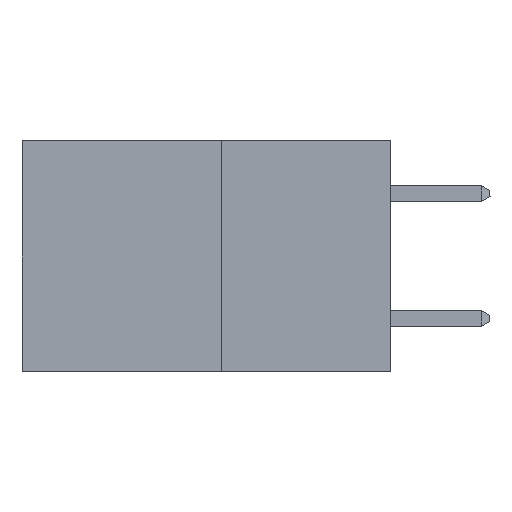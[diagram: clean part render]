
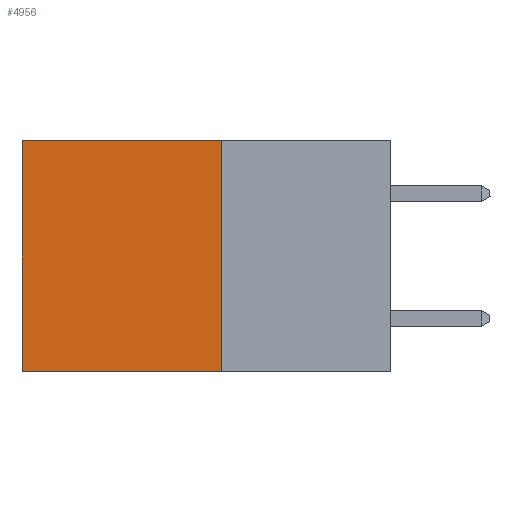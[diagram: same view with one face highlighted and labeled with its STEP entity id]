
A CAD part, left-side view. The second image highlights one B-rep face of the part: STEP entity #4956.
In plain terms, the highlighted planar face has unit normal (-1, 0, 0).
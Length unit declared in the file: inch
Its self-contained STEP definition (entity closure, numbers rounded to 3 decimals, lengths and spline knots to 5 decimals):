
#220 = LINE ( 'NONE', #9348, #20067 ) ;
#1047 = EDGE_CURVE ( 'NONE', #11600, #29045, #3526, .T. ) ;
#1293 = CARTESIAN_POINT ( 'NONE',  ( 0.277, 0.59, 0. ) ) ;
#1620 = PLANE ( 'NONE',  #19082 ) ;
#2079 = EDGE_LOOP ( 'NONE', ( #10348, #6432, #28435, #22410 ) ) ;
#3028 = CARTESIAN_POINT ( 'NONE',  ( 0.277, 0.27, -0.37 ) ) ;
#3526 = LINE ( 'NONE', #19468, #16709 ) ;
#4143 = DIRECTION ( 'NONE',  ( 0., 0., -1. ) ) ;
#4956 = ADVANCED_FACE ( 'NONE', ( #31731 ), #1620, .F. ) ;
#5310 = LINE ( 'NONE', #24060, #17729 ) ;
#6432 = ORIENTED_EDGE ( 'NONE', *, *, #1047, .F. ) ;
#6723 = CARTESIAN_POINT ( 'NONE',  ( 0.277, 0.59, -0.37 ) ) ;
#9348 = CARTESIAN_POINT ( 'NONE',  ( 0.277, 0.27, -0.37 ) ) ;
#10348 = ORIENTED_EDGE ( 'NONE', *, *, #30693, .T. ) ;
#11600 = VERTEX_POINT ( 'NONE', #3028 ) ;
#16155 = CARTESIAN_POINT ( 'NONE',  ( 0.277, 0.27, 0. ) ) ;
#16709 = VECTOR ( 'NONE', #31703, 39.37008 ) ;
#17137 = CARTESIAN_POINT ( 'NONE',  ( 0.277, 0.59, -0.37 ) ) ;
#17714 = LINE ( 'NONE', #17137, #29440 ) ;
#17729 = VECTOR ( 'NONE', #31633, 39.37008 ) ;
#19017 = DIRECTION ( 'NONE',  ( 1., 0., 0. ) ) ;
#19082 = AXIS2_PLACEMENT_3D ( 'NONE', #26446, #19017, #4143 ) ;
#19208 = DIRECTION ( 'NONE',  ( 0., 0., -1. ) ) ;
#19468 = CARTESIAN_POINT ( 'NONE',  ( 0.277, 0.27, -0.37 ) ) ;
#19660 = DIRECTION ( 'NONE',  ( 0., 0., -1. ) ) ;
#20067 = VECTOR ( 'NONE', #19208, 39.37008 ) ;
#21443 = VERTEX_POINT ( 'NONE', #1293 ) ;
#22150 = VERTEX_POINT ( 'NONE', #16155 ) ;
#22410 = ORIENTED_EDGE ( 'NONE', *, *, #31249, .T. ) ;
#24060 = CARTESIAN_POINT ( 'NONE',  ( 0.277, 0.27, 0. ) ) ;
#26446 = CARTESIAN_POINT ( 'NONE',  ( 0.277, 0.27, -0.37 ) ) ;
#28435 = ORIENTED_EDGE ( 'NONE', *, *, #30573, .F. ) ;
#29045 = VERTEX_POINT ( 'NONE', #6723 ) ;
#29440 = VECTOR ( 'NONE', #19660, 39.37008 ) ;
#30573 = EDGE_CURVE ( 'NONE', #22150, #11600, #220, .T. ) ;
#30693 = EDGE_CURVE ( 'NONE', #21443, #29045, #17714, .T. ) ;
#31249 = EDGE_CURVE ( 'NONE', #22150, #21443, #5310, .T. ) ;
#31633 = DIRECTION ( 'NONE',  ( 0., 1., 0. ) ) ;
#31703 = DIRECTION ( 'NONE',  ( 0., 1., 0. ) ) ;
#31731 = FACE_OUTER_BOUND ( 'NONE', #2079, .T. ) ;
